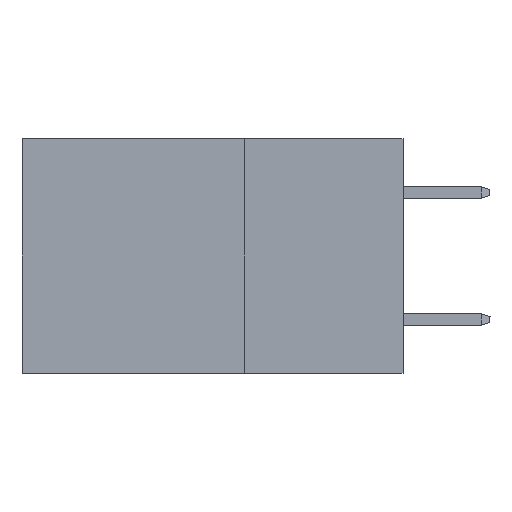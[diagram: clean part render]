
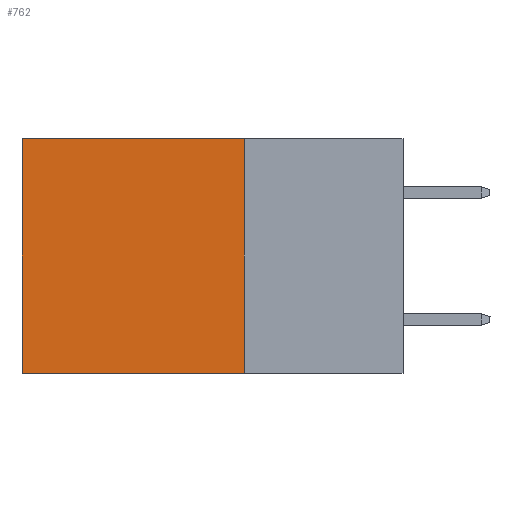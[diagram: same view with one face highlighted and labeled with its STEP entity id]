
A CAD part, left-side view. The second image highlights one B-rep face of the part: STEP entity #762.
In plain terms, the highlighted planar face has unit normal (-1, 0, 0).
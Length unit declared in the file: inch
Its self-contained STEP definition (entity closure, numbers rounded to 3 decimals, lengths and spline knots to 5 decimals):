
#35 = LINE ( 'NONE', #6794, #8338 ) ;
#525 = EDGE_CURVE ( 'NONE', #12469, #2182, #9573, .T. ) ;
#614 = EDGE_CURVE ( 'NONE', #11892, #12469, #35, .T. ) ;
#762 = ADVANCED_FACE ( 'NONE', ( #16510 ), #19732, .F. ) ;
#1272 = DIRECTION ( 'NONE',  ( 0., 0., -1. ) ) ;
#2182 = VERTEX_POINT ( 'NONE', #14829 ) ;
#2529 = CARTESIAN_POINT ( 'NONE',  ( 0.2875, 0.6, 0. ) ) ;
#4029 = CARTESIAN_POINT ( 'NONE',  ( 0.2875, 0.25, 0. ) ) ;
#6202 = ORIENTED_EDGE ( 'NONE', *, *, #7414, .F. ) ;
#6584 = VECTOR ( 'NONE', #1272, 39.37008 ) ;
#6794 = CARTESIAN_POINT ( 'NONE',  ( 0.2875, 0.25, 0. ) ) ;
#7414 = EDGE_CURVE ( 'NONE', #17447, #2182, #16518, .T. ) ;
#7761 = DIRECTION ( 'NONE',  ( 1., 0., 0. ) ) ;
#7797 = DIRECTION ( 'NONE',  ( 0., 0., -1. ) ) ;
#8338 = VECTOR ( 'NONE', #11999, 39.37008 ) ;
#9573 = LINE ( 'NONE', #11350, #6584 ) ;
#9670 = CARTESIAN_POINT ( 'NONE',  ( 0.2875, 0.25, 0. ) ) ;
#9821 = ORIENTED_EDGE ( 'NONE', *, *, #614, .T. ) ;
#11350 = CARTESIAN_POINT ( 'NONE',  ( 0.2875, 0.6, 0. ) ) ;
#11696 = EDGE_CURVE ( 'NONE', #11892, #17447, #17986, .T. ) ;
#11892 = VERTEX_POINT ( 'NONE', #20719 ) ;
#11999 = DIRECTION ( 'NONE',  ( 0., 1., 0. ) ) ;
#12206 = ORIENTED_EDGE ( 'NONE', *, *, #525, .T. ) ;
#12469 = VERTEX_POINT ( 'NONE', #2529 ) ;
#14202 = CARTESIAN_POINT ( 'NONE',  ( 0.2875, 0.25, -0.37 ) ) ;
#14829 = CARTESIAN_POINT ( 'NONE',  ( 0.2875, 0.6, -0.37 ) ) ;
#15301 = EDGE_LOOP ( 'NONE', ( #12206, #6202, #20947, #9821 ) ) ;
#16412 = CARTESIAN_POINT ( 'NONE',  ( 0.2875, 0.25, -0.37 ) ) ;
#16510 = FACE_OUTER_BOUND ( 'NONE', #15301, .T. ) ;
#16518 = LINE ( 'NONE', #16412, #18424 ) ;
#17447 = VERTEX_POINT ( 'NONE', #14202 ) ;
#17548 = AXIS2_PLACEMENT_3D ( 'NONE', #4029, #7761, #17842 ) ;
#17842 = DIRECTION ( 'NONE',  ( 0., 0., -1. ) ) ;
#17986 = LINE ( 'NONE', #9670, #19656 ) ;
#18424 = VECTOR ( 'NONE', #21508, 39.37008 ) ;
#19656 = VECTOR ( 'NONE', #7797, 39.37008 ) ;
#19732 = PLANE ( 'NONE',  #17548 ) ;
#20719 = CARTESIAN_POINT ( 'NONE',  ( 0.2875, 0.25, 0. ) ) ;
#20947 = ORIENTED_EDGE ( 'NONE', *, *, #11696, .F. ) ;
#21508 = DIRECTION ( 'NONE',  ( 0., 1., 0. ) ) ;
